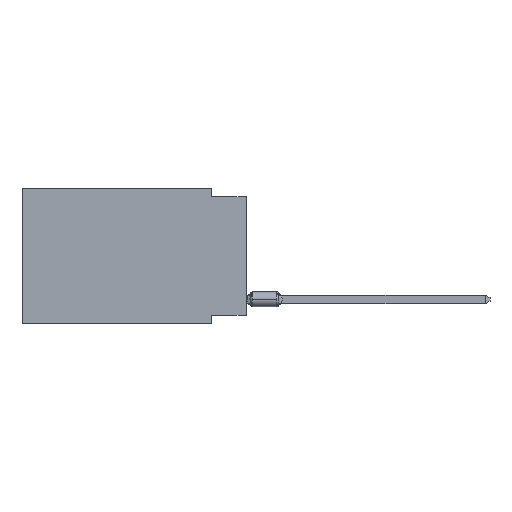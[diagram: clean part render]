
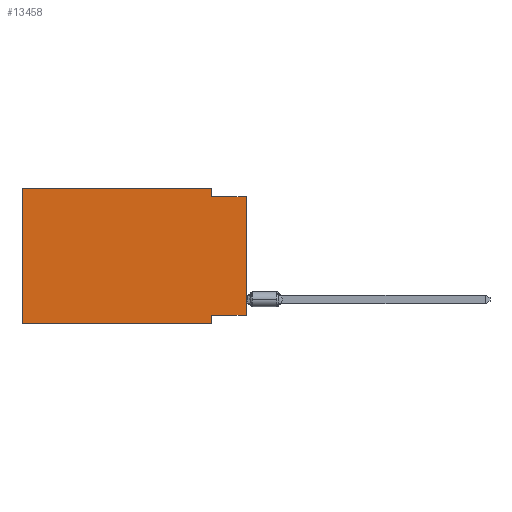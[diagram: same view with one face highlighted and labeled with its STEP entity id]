
A CAD part, left-side view. The second image highlights one B-rep face of the part: STEP entity #13458.
In plain terms, the highlighted planar face has unit normal (-1, 0, 0).
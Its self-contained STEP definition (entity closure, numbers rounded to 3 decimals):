
#315 = CARTESIAN_POINT ( 'NONE',  ( 0., 16.383, 0. ) ) ;
#499 = EDGE_CURVE ( 'NONE', #9376, #16129, #6955, .T. ) ;
#1844 = EDGE_CURVE ( 'NONE', #19080, #17498, #11477, .T. ) ;
#2202 = CARTESIAN_POINT ( 'NONE',  ( 0., 16.383, 0. ) ) ;
#2204 = DIRECTION ( 'NONE',  ( 1., 0., 0. ) ) ;
#2250 = LINE ( 'NONE', #18831, #13158 ) ;
#2557 = AXIS2_PLACEMENT_3D ( 'NONE', #315, #2204, #6579 ) ;
#2788 = ORIENTED_EDGE ( 'NONE', *, *, #5378, .F. ) ;
#2886 = VECTOR ( 'NONE', #14656, 1000. ) ;
#2936 = CARTESIAN_POINT ( 'NONE',  ( 0., 16.383, 0. ) ) ;
#2970 = VECTOR ( 'NONE', #15721, 1000. ) ;
#3331 = ORIENTED_EDGE ( 'NONE', *, *, #5096, .F. ) ;
#3599 = VECTOR ( 'NONE', #12126, 1000. ) ;
#3738 = EDGE_CURVE ( 'NONE', #16129, #16932, #11928, .T. ) ;
#4185 = LINE ( 'NONE', #10242, #3599 ) ;
#5096 = EDGE_CURVE ( 'NONE', #17870, #14127, #19340, .T. ) ;
#5210 = CARTESIAN_POINT ( 'NONE',  ( 0., 0., -9.271 ) ) ;
#5378 = EDGE_CURVE ( 'NONE', #19080, #9376, #13371, .T. ) ;
#5850 = CARTESIAN_POINT ( 'NONE',  ( 0., 2.54, 0. ) ) ;
#5979 = CARTESIAN_POINT ( 'NONE',  ( 0., 0., -0.635 ) ) ;
#6579 = DIRECTION ( 'NONE',  ( 0., 0., -1. ) ) ;
#6955 = LINE ( 'NONE', #2202, #2970 ) ;
#6988 = VECTOR ( 'NONE', #9124, 1000. ) ;
#7356 = LINE ( 'NONE', #16300, #7605 ) ;
#7605 = VECTOR ( 'NONE', #11544, 1000. ) ;
#7792 = CARTESIAN_POINT ( 'NONE',  ( 0., 16.383, 0. ) ) ;
#8174 = FACE_OUTER_BOUND ( 'NONE', #17728, .T. ) ;
#8297 = EDGE_CURVE ( 'NONE', #17870, #10924, #4185, .T. ) ;
#9011 = VECTOR ( 'NONE', #14833, 1000. ) ;
#9124 = DIRECTION ( 'NONE',  ( 0., 1., 0. ) ) ;
#9376 = VERTEX_POINT ( 'NONE', #7792 ) ;
#9795 = DIRECTION ( 'NONE',  ( 0., 0., -1. ) ) ;
#10204 = ORIENTED_EDGE ( 'NONE', *, *, #1844, .T. ) ;
#10242 = CARTESIAN_POINT ( 'NONE',  ( 0., 0., 0. ) ) ;
#10924 = VERTEX_POINT ( 'NONE', #5979 ) ;
#11266 = EDGE_CURVE ( 'NONE', #16932, #10924, #7356, .T. ) ;
#11477 = LINE ( 'NONE', #13161, #9011 ) ;
#11544 = DIRECTION ( 'NONE',  ( 0., -1., 0. ) ) ;
#11928 = LINE ( 'NONE', #5850, #14033 ) ;
#12126 = DIRECTION ( 'NONE',  ( 0., 0., 1. ) ) ;
#12786 = CARTESIAN_POINT ( 'NONE',  ( 0., 2.54, -9.906 ) ) ;
#12801 = ORIENTED_EDGE ( 'NONE', *, *, #8297, .T. ) ;
#12899 = ORIENTED_EDGE ( 'NONE', *, *, #11266, .F. ) ;
#13158 = VECTOR ( 'NONE', #9795, 1000. ) ;
#13161 = CARTESIAN_POINT ( 'NONE',  ( 0., 16.383, -9.906 ) ) ;
#13371 = LINE ( 'NONE', #2936, #2886 ) ;
#13458 = ADVANCED_FACE ( 'NONE', ( #8174 ), #14225, .F. ) ;
#13971 = CARTESIAN_POINT ( 'NONE',  ( 0., 2.54, 0. ) ) ;
#14033 = VECTOR ( 'NONE', #14875, 1000. ) ;
#14127 = VERTEX_POINT ( 'NONE', #15091 ) ;
#14225 = PLANE ( 'NONE',  #2557 ) ;
#14656 = DIRECTION ( 'NONE',  ( 0., 0., 1. ) ) ;
#14833 = DIRECTION ( 'NONE',  ( 0., -1., 0. ) ) ;
#14875 = DIRECTION ( 'NONE',  ( 0., 0., -1. ) ) ;
#15091 = CARTESIAN_POINT ( 'NONE',  ( 0., 2.54, -9.271 ) ) ;
#15721 = DIRECTION ( 'NONE',  ( 0., -1., 0. ) ) ;
#16129 = VERTEX_POINT ( 'NONE', #13971 ) ;
#16300 = CARTESIAN_POINT ( 'NONE',  ( 0., 0., -0.635 ) ) ;
#16439 = ORIENTED_EDGE ( 'NONE', *, *, #3738, .F. ) ;
#16503 = ORIENTED_EDGE ( 'NONE', *, *, #17501, .F. ) ;
#16932 = VERTEX_POINT ( 'NONE', #18854 ) ;
#17498 = VERTEX_POINT ( 'NONE', #12786 ) ;
#17501 = EDGE_CURVE ( 'NONE', #14127, #17498, #2250, .T. ) ;
#17728 = EDGE_LOOP ( 'NONE', ( #12801, #12899, #16439, #17895, #2788, #10204, #16503, #3331 ) ) ;
#17853 = CARTESIAN_POINT ( 'NONE',  ( 0., 0., -9.271 ) ) ;
#17870 = VERTEX_POINT ( 'NONE', #5210 ) ;
#17895 = ORIENTED_EDGE ( 'NONE', *, *, #499, .F. ) ;
#18670 = CARTESIAN_POINT ( 'NONE',  ( 0., 16.383, -9.906 ) ) ;
#18831 = CARTESIAN_POINT ( 'NONE',  ( 0., 2.54, -9.906 ) ) ;
#18854 = CARTESIAN_POINT ( 'NONE',  ( 0., 2.54, -0.635 ) ) ;
#19080 = VERTEX_POINT ( 'NONE', #18670 ) ;
#19340 = LINE ( 'NONE', #17853, #6988 ) ;
